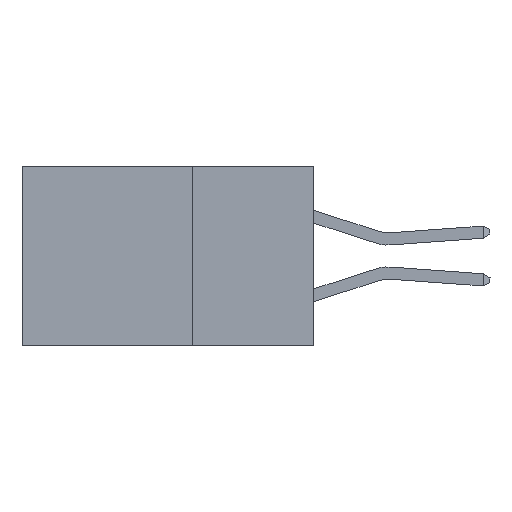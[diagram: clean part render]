
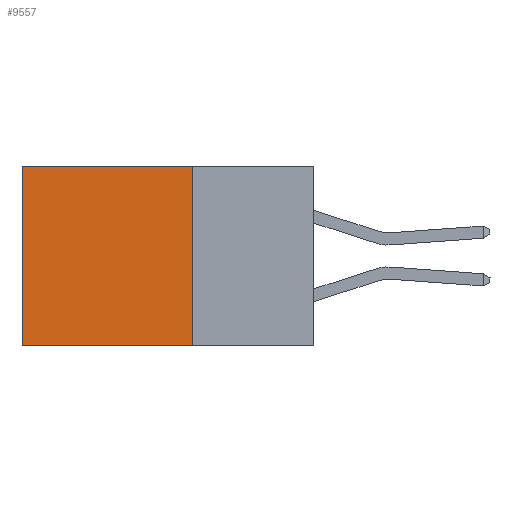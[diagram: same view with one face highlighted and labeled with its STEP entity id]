
A CAD part, left-side view. The second image highlights one B-rep face of the part: STEP entity #9557.
In plain terms, the highlighted planar face has unit normal (-1, 0, 0).
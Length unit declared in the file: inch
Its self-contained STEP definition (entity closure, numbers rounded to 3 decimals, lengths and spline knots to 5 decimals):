
#73 = ORIENTED_EDGE ( 'NONE', *, *, #20208, .T. ) ;
#1289 = VECTOR ( 'NONE', #12086, 39.37008 ) ;
#1318 = ORIENTED_EDGE ( 'NONE', *, *, #42044, .T. ) ;
#2641 = CARTESIAN_POINT ( 'NONE',  ( 0.2875, 0.25, -0.37 ) ) ;
#6316 = ORIENTED_EDGE ( 'NONE', *, *, #35202, .F. ) ;
#7725 = LINE ( 'NONE', #42730, #23638 ) ;
#7985 = EDGE_LOOP ( 'NONE', ( #73, #38880, #6316, #1318 ) ) ;
#8134 = EDGE_CURVE ( 'NONE', #24460, #9765, #7725, .T. ) ;
#9557 = ADVANCED_FACE ( 'NONE', ( #17100 ), #13527, .F. ) ;
#9562 = VECTOR ( 'NONE', #42496, 39.37008 ) ;
#9765 = VERTEX_POINT ( 'NONE', #34605 ) ;
#11819 = CARTESIAN_POINT ( 'NONE',  ( 0.2875, 0.25, 0. ) ) ;
#12086 = DIRECTION ( 'NONE',  ( 0., 0., -1. ) ) ;
#13527 = PLANE ( 'NONE',  #28431 ) ;
#15137 = CARTESIAN_POINT ( 'NONE',  ( 0.2875, 0.6, 0. ) ) ;
#17100 = FACE_OUTER_BOUND ( 'NONE', #7985, .T. ) ;
#17475 = LINE ( 'NONE', #11819, #9562 ) ;
#20208 = EDGE_CURVE ( 'NONE', #41465, #9765, #25754, .T. ) ;
#20334 = DIRECTION ( 'NONE',  ( 0., 1., 0. ) ) ;
#21546 = VERTEX_POINT ( 'NONE', #26728 ) ;
#23638 = VECTOR ( 'NONE', #32363, 39.37008 ) ;
#24038 = LINE ( 'NONE', #36417, #43176 ) ;
#24460 = VERTEX_POINT ( 'NONE', #2641 ) ;
#25754 = LINE ( 'NONE', #15137, #1289 ) ;
#26728 = CARTESIAN_POINT ( 'NONE',  ( 0.2875, 0.25, 0. ) ) ;
#28431 = AXIS2_PLACEMENT_3D ( 'NONE', #33882, #37151, #37295 ) ;
#32363 = DIRECTION ( 'NONE',  ( 0., 1., 0. ) ) ;
#33882 = CARTESIAN_POINT ( 'NONE',  ( 0.2875, 0.25, 0. ) ) ;
#34605 = CARTESIAN_POINT ( 'NONE',  ( 0.2875, 0.6, -0.37 ) ) ;
#35202 = EDGE_CURVE ( 'NONE', #21546, #24460, #17475, .T. ) ;
#36417 = CARTESIAN_POINT ( 'NONE',  ( 0.2875, 0.25, 0. ) ) ;
#36773 = CARTESIAN_POINT ( 'NONE',  ( 0.2875, 0.6, 0. ) ) ;
#37151 = DIRECTION ( 'NONE',  ( 1., 0., 0. ) ) ;
#37295 = DIRECTION ( 'NONE',  ( 0., 0., -1. ) ) ;
#38880 = ORIENTED_EDGE ( 'NONE', *, *, #8134, .F. ) ;
#41465 = VERTEX_POINT ( 'NONE', #36773 ) ;
#42044 = EDGE_CURVE ( 'NONE', #21546, #41465, #24038, .T. ) ;
#42496 = DIRECTION ( 'NONE',  ( 0., 0., -1. ) ) ;
#42730 = CARTESIAN_POINT ( 'NONE',  ( 0.2875, 0.25, -0.37 ) ) ;
#43176 = VECTOR ( 'NONE', #20334, 39.37008 ) ;
